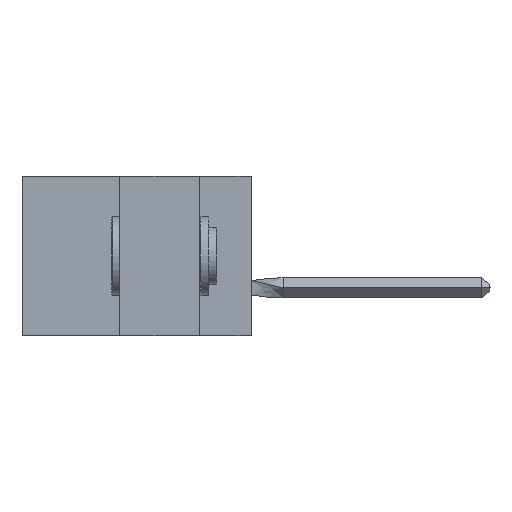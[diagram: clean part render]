
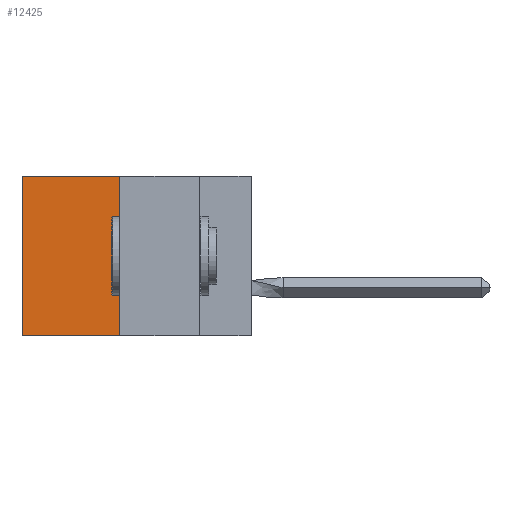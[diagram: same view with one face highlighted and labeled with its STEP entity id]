
A CAD part, left-side view. The second image highlights one B-rep face of the part: STEP entity #12425.
In plain terms, the highlighted planar face has unit normal (-1, 0, 0).
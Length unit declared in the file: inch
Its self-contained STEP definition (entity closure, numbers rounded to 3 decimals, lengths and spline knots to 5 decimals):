
#81 = EDGE_CURVE ( 'NONE', #22618, #28344, #18553, .T. ) ;
#517 = VERTEX_POINT ( 'NONE', #21469 ) ;
#569 = VECTOR ( 'NONE', #1251, 39.37008 ) ;
#699 = VECTOR ( 'NONE', #8751, 39.37008 ) ;
#1251 = DIRECTION ( 'NONE',  ( 0., 1., 0. ) ) ;
#1813 = AXIS2_PLACEMENT_3D ( 'NONE', #6529, #24468, #18040 ) ;
#4305 = PLANE ( 'NONE',  #1813 ) ;
#4954 = LINE ( 'NONE', #26093, #6353 ) ;
#6353 = VECTOR ( 'NONE', #28286, 39.37008 ) ;
#6529 = CARTESIAN_POINT ( 'NONE',  ( 0.305, 0.413, -0.5 ) ) ;
#6841 = CARTESIAN_POINT ( 'NONE',  ( 0.305, 0.413, 0. ) ) ;
#6916 = FACE_OUTER_BOUND ( 'NONE', #10316, .T. ) ;
#8385 = EDGE_CURVE ( 'NONE', #28344, #17425, #23320, .T. ) ;
#8751 = DIRECTION ( 'NONE',  ( 0., 1., 0. ) ) ;
#9825 = CARTESIAN_POINT ( 'NONE',  ( 0.305, 0.72, -0.5 ) ) ;
#10316 = EDGE_LOOP ( 'NONE', ( #15902, #22141, #27438, #27445 ) ) ;
#12425 = ADVANCED_FACE ( 'NONE', ( #6916 ), #4305, .F. ) ;
#15173 = CARTESIAN_POINT ( 'NONE',  ( 0.305, 0.413, 0. ) ) ;
#15843 = CARTESIAN_POINT ( 'NONE',  ( 0.305, 0.72, 0. ) ) ;
#15902 = ORIENTED_EDGE ( 'NONE', *, *, #8385, .T. ) ;
#17425 = VERTEX_POINT ( 'NONE', #9825 ) ;
#18040 = DIRECTION ( 'NONE',  ( 0., 0., -1. ) ) ;
#18231 = CARTESIAN_POINT ( 'NONE',  ( 0.305, 0.72, -0.5 ) ) ;
#18553 = LINE ( 'NONE', #15173, #699 ) ;
#19410 = EDGE_CURVE ( 'NONE', #517, #17425, #26986, .T. ) ;
#20922 = CARTESIAN_POINT ( 'NONE',  ( 0.305, 0.413, -0.5 ) ) ;
#21392 = EDGE_CURVE ( 'NONE', #22618, #517, #4954, .T. ) ;
#21469 = CARTESIAN_POINT ( 'NONE',  ( 0.305, 0.413, -0.5 ) ) ;
#22141 = ORIENTED_EDGE ( 'NONE', *, *, #19410, .F. ) ;
#22618 = VERTEX_POINT ( 'NONE', #6841 ) ;
#22954 = VECTOR ( 'NONE', #26945, 39.37008 ) ;
#23320 = LINE ( 'NONE', #18231, #22954 ) ;
#24468 = DIRECTION ( 'NONE',  ( 1., 0., 0. ) ) ;
#26093 = CARTESIAN_POINT ( 'NONE',  ( 0.305, 0.413, -0.5 ) ) ;
#26945 = DIRECTION ( 'NONE',  ( 0., 0., -1. ) ) ;
#26986 = LINE ( 'NONE', #20922, #569 ) ;
#27438 = ORIENTED_EDGE ( 'NONE', *, *, #21392, .F. ) ;
#27445 = ORIENTED_EDGE ( 'NONE', *, *, #81, .T. ) ;
#28286 = DIRECTION ( 'NONE',  ( 0., 0., -1. ) ) ;
#28344 = VERTEX_POINT ( 'NONE', #15843 ) ;
